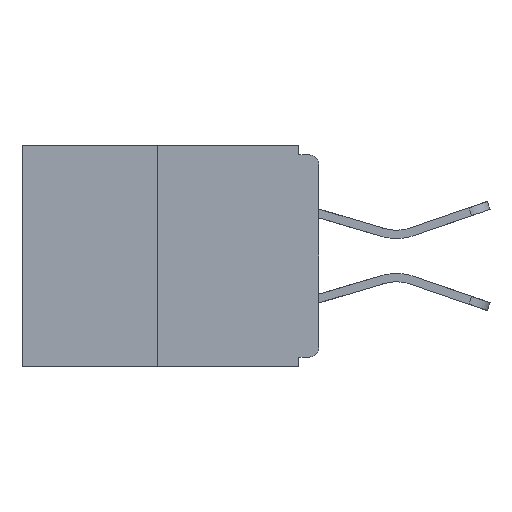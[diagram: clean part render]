
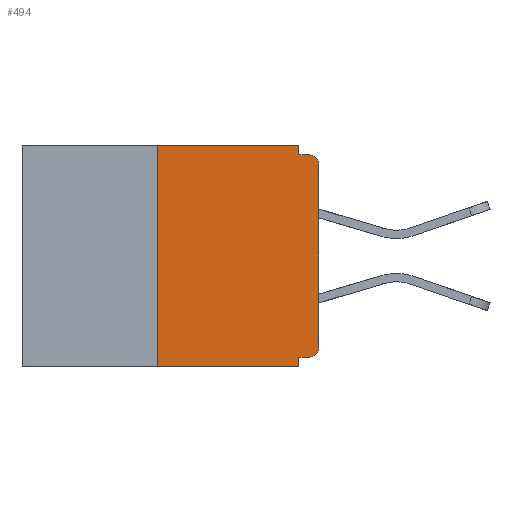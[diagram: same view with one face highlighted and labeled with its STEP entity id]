
A CAD part, left-side view. The second image highlights one B-rep face of the part: STEP entity #494.
In plain terms, the highlighted planar face has unit normal (-1, 0, 0).
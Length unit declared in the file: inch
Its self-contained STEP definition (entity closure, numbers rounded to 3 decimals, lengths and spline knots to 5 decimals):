
#220 = CARTESIAN_POINT ( 'NONE',  ( 0., 0.46, 0. ) ) ;
#494 = ADVANCED_FACE ( 'NONE', ( #2455 ), #1825, .F. ) ;
#963 = CARTESIAN_POINT ( 'NONE',  ( 0., 0.031, -0.328 ) ) ;
#1033 = CARTESIAN_POINT ( 'NONE',  ( 0., 0., -0.328 ) ) ;
#1219 = DIRECTION ( 'NONE',  ( -1., 0., 0. ) ) ;
#1377 = DIRECTION ( 'NONE',  ( -1., 0., 0. ) ) ;
#1752 = EDGE_CURVE ( 'NONE', #4093, #9833, #28251, .T. ) ;
#1825 = PLANE ( 'NONE',  #7372 ) ;
#1840 = VECTOR ( 'NONE', #11959, 39.37008 ) ;
#1998 = VECTOR ( 'NONE', #25535, 39.37008 ) ;
#2455 = FACE_OUTER_BOUND ( 'NONE', #28056, .T. ) ;
#2836 = ORIENTED_EDGE ( 'NONE', *, *, #12383, .T. ) ;
#3024 = CARTESIAN_POINT ( 'NONE',  ( 0., 0.25, 0. ) ) ;
#3536 = CARTESIAN_POINT ( 'NONE',  ( 0., 0., -0.015 ) ) ;
#4093 = VERTEX_POINT ( 'NONE', #22126 ) ;
#4161 = AXIS2_PLACEMENT_3D ( 'NONE', #30341, #1377, #20694 ) ;
#4265 = CARTESIAN_POINT ( 'NONE',  ( 0., 0.015, -0.328 ) ) ;
#5511 = VECTOR ( 'NONE', #17423, 39.37008 ) ;
#5994 = CARTESIAN_POINT ( 'NONE',  ( 0., 0.031, -0.343 ) ) ;
#6138 = VECTOR ( 'NONE', #8532, 39.37008 ) ;
#6688 = LINE ( 'NONE', #28959, #17391 ) ;
#7002 = ORIENTED_EDGE ( 'NONE', *, *, #20672, .F. ) ;
#7062 = DIRECTION ( 'NONE',  ( 0., -1., 0. ) ) ;
#7372 = AXIS2_PLACEMENT_3D ( 'NONE', #220, #20075, #22742 ) ;
#7393 = VERTEX_POINT ( 'NONE', #30969 ) ;
#7518 = EDGE_CURVE ( 'NONE', #4093, #20302, #12600, .T. ) ;
#7674 = CARTESIAN_POINT ( 'NONE',  ( 0., 0., -0.03 ) ) ;
#8189 = DIRECTION ( 'NONE',  ( 0., 0., -1. ) ) ;
#8425 = DIRECTION ( 'NONE',  ( 0., 0., -1. ) ) ;
#8532 = DIRECTION ( 'NONE',  ( 0., 0., 1. ) ) ;
#9208 = CARTESIAN_POINT ( 'NONE',  ( 0., 0.46, -0.343 ) ) ;
#9833 = VERTEX_POINT ( 'NONE', #15483 ) ;
#10935 = ORIENTED_EDGE ( 'NONE', *, *, #7518, .F. ) ;
#11170 = VERTEX_POINT ( 'NONE', #963 ) ;
#11213 = ORIENTED_EDGE ( 'NONE', *, *, #17276, .F. ) ;
#11673 = DIRECTION ( 'NONE',  ( 0., -1., 0. ) ) ;
#11959 = DIRECTION ( 'NONE',  ( 0., 0., 1. ) ) ;
#12159 = CARTESIAN_POINT ( 'NONE',  ( 0., 0.031, 0. ) ) ;
#12383 = EDGE_CURVE ( 'NONE', #28358, #7393, #30336, .T. ) ;
#12567 = VECTOR ( 'NONE', #11673, 39.37008 ) ;
#12600 = LINE ( 'NONE', #13680, #6138 ) ;
#12914 = CARTESIAN_POINT ( 'NONE',  ( 0., 0., -0.313 ) ) ;
#13680 = CARTESIAN_POINT ( 'NONE',  ( 0., 0.25, 0. ) ) ;
#14430 = VERTEX_POINT ( 'NONE', #12914 ) ;
#14475 = ORIENTED_EDGE ( 'NONE', *, *, #18822, .F. ) ;
#15483 = CARTESIAN_POINT ( 'NONE',  ( 0., 0.031, -0.343 ) ) ;
#15619 = LINE ( 'NONE', #19297, #1840 ) ;
#16037 = VERTEX_POINT ( 'NONE', #26267 ) ;
#17276 = EDGE_CURVE ( 'NONE', #23230, #7393, #26485, .T. ) ;
#17391 = VECTOR ( 'NONE', #7062, 39.37008 ) ;
#17423 = DIRECTION ( 'NONE',  ( 0., 0., -1. ) ) ;
#18181 = DIRECTION ( 'NONE',  ( 0., 1., 0. ) ) ;
#18450 = ORIENTED_EDGE ( 'NONE', *, *, #1752, .T. ) ;
#18822 = EDGE_CURVE ( 'NONE', #11170, #9833, #26756, .T. ) ;
#19297 = CARTESIAN_POINT ( 'NONE',  ( 0., 0., 0. ) ) ;
#19369 = EDGE_CURVE ( 'NONE', #14430, #28358, #15619, .T. ) ;
#19400 = CIRCLE ( 'NONE', #24695, 0.015 ) ;
#20075 = DIRECTION ( 'NONE',  ( 1., 0., 0. ) ) ;
#20302 = VERTEX_POINT ( 'NONE', #3024 ) ;
#20672 = EDGE_CURVE ( 'NONE', #28701, #11170, #22101, .T. ) ;
#20694 = DIRECTION ( 'NONE',  ( 0., 0., -1. ) ) ;
#21653 = EDGE_CURVE ( 'NONE', #20302, #16037, #6688, .T. ) ;
#21798 = CARTESIAN_POINT ( 'NONE',  ( 0., 0.031, -0.015 ) ) ;
#22101 = LINE ( 'NONE', #1033, #24363 ) ;
#22126 = CARTESIAN_POINT ( 'NONE',  ( 0., 0.25, -0.343 ) ) ;
#22742 = DIRECTION ( 'NONE',  ( 0., 0., -1. ) ) ;
#23230 = VERTEX_POINT ( 'NONE', #21798 ) ;
#24363 = VECTOR ( 'NONE', #18181, 39.37008 ) ;
#24695 = AXIS2_PLACEMENT_3D ( 'NONE', #25286, #1219, #8189 ) ;
#24982 = LINE ( 'NONE', #12159, #5511 ) ;
#25286 = CARTESIAN_POINT ( 'NONE',  ( 0., 0.015, -0.313 ) ) ;
#25535 = DIRECTION ( 'NONE',  ( 0., -1., 0. ) ) ;
#26123 = ORIENTED_EDGE ( 'NONE', *, *, #19369, .T. ) ;
#26267 = CARTESIAN_POINT ( 'NONE',  ( 0., 0.031, 0. ) ) ;
#26385 = VECTOR ( 'NONE', #8425, 39.37008 ) ;
#26485 = LINE ( 'NONE', #3536, #1998 ) ;
#26540 = EDGE_CURVE ( 'NONE', #28701, #14430, #19400, .T. ) ;
#26756 = LINE ( 'NONE', #5994, #26385 ) ;
#27506 = ORIENTED_EDGE ( 'NONE', *, *, #26540, .T. ) ;
#27868 = ORIENTED_EDGE ( 'NONE', *, *, #21653, .F. ) ;
#28056 = EDGE_LOOP ( 'NONE', ( #27868, #10935, #18450, #14475, #7002, #27506, #26123, #2836, #11213, #31078 ) ) ;
#28213 = EDGE_CURVE ( 'NONE', #16037, #23230, #24982, .T. ) ;
#28251 = LINE ( 'NONE', #9208, #12567 ) ;
#28358 = VERTEX_POINT ( 'NONE', #7674 ) ;
#28701 = VERTEX_POINT ( 'NONE', #4265 ) ;
#28959 = CARTESIAN_POINT ( 'NONE',  ( 0., 0.46, 0. ) ) ;
#30336 = CIRCLE ( 'NONE', #4161, 0.015 ) ;
#30341 = CARTESIAN_POINT ( 'NONE',  ( 0., 0.015, -0.03 ) ) ;
#30969 = CARTESIAN_POINT ( 'NONE',  ( 0., 0.015, -0.015 ) ) ;
#31078 = ORIENTED_EDGE ( 'NONE', *, *, #28213, .F. ) ;
